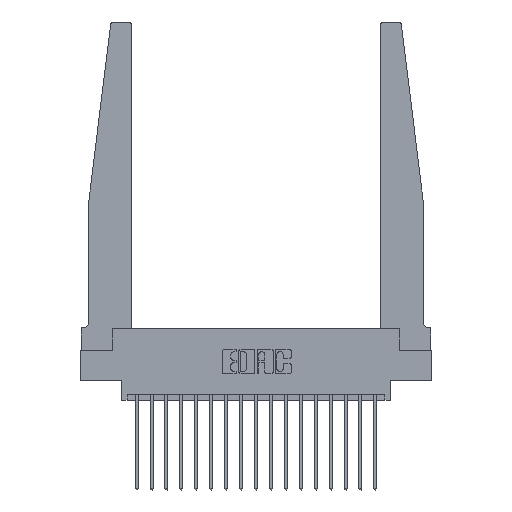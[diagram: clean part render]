
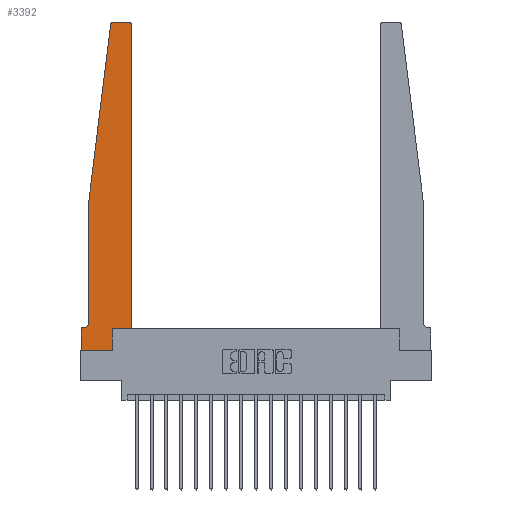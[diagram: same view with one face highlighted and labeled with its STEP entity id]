
A CAD part, top view. The second image highlights one B-rep face of the part: STEP entity #3392.
In plain terms, the highlighted planar face has unit normal (0, 0, 1).
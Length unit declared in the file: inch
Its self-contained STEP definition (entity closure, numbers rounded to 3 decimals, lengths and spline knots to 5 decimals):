
#1297 = DIRECTION ( 'NONE',  ( 0., 0., -1. ) ) ;
#1470 = VERTEX_POINT ( 'NONE', #15704 ) ;
#1640 = VECTOR ( 'NONE', #2279, 39.37008 ) ;
#1730 = DIRECTION ( 'NONE',  ( 0., 0., 1. ) ) ;
#1853 = CARTESIAN_POINT ( 'NONE',  ( 0.425, 2.72, 0.37 ) ) ;
#1882 = CARTESIAN_POINT ( 'NONE',  ( 0.24675, 2.72367, 0.37 ) ) ;
#1940 = CIRCLE ( 'NONE', #12543, 0.03 ) ;
#2054 = LINE ( 'NONE', #3768, #9599 ) ;
#2268 = CARTESIAN_POINT ( 'NONE',  ( 0.25, 2.75, 0.37 ) ) ;
#2279 = DIRECTION ( 'NONE',  ( 0., -1., 0. ) ) ;
#2594 = CARTESIAN_POINT ( 'NONE',  ( 0.015, 0.2375, 0.37 ) ) ;
#3093 = ORIENTED_EDGE ( 'NONE', *, *, #6055, .T. ) ;
#3392 = ADVANCED_FACE ( 'NONE', ( #4985 ), #8127, .T. ) ;
#3506 = LINE ( 'NONE', #9547, #18701 ) ;
#3515 = ORIENTED_EDGE ( 'NONE', *, *, #8881, .T. ) ;
#3593 = ORIENTED_EDGE ( 'NONE', *, *, #10420, .T. ) ;
#3768 = CARTESIAN_POINT ( 'NONE',  ( 0.065, 1.25, 0.37 ) ) ;
#3880 = ORIENTED_EDGE ( 'NONE', *, *, #8476, .T. ) ;
#3957 = ORIENTED_EDGE ( 'NONE', *, *, #13938, .T. ) ;
#4154 = LINE ( 'NONE', #19502, #17698 ) ;
#4369 = VECTOR ( 'NONE', #11641, 39.37008 ) ;
#4474 = AXIS2_PLACEMENT_3D ( 'NONE', #18731, #5181, #8225 ) ;
#4568 = EDGE_CURVE ( 'NONE', #5965, #17212, #12161, .T. ) ;
#4656 = DIRECTION ( 'NONE',  ( 1., 0., 0. ) ) ;
#4985 = FACE_OUTER_BOUND ( 'NONE', #17135, .T. ) ;
#5181 = DIRECTION ( 'NONE',  ( 0., 0., 1. ) ) ;
#5259 = VECTOR ( 'NONE', #18855, 39.37008 ) ;
#5777 = EDGE_CURVE ( 'NONE', #17212, #12050, #10070, .T. ) ;
#5862 = EDGE_CURVE ( 'NONE', #6694, #8320, #12257, .T. ) ;
#5960 = DIRECTION ( 'NONE',  ( 0., 1., 0. ) ) ;
#5965 = VERTEX_POINT ( 'NONE', #16452 ) ;
#6055 = EDGE_CURVE ( 'NONE', #19147, #15143, #11442, .T. ) ;
#6057 = VERTEX_POINT ( 'NONE', #19154 ) ;
#6172 = CARTESIAN_POINT ( 'NONE',  ( 0.27653, 2.72, 0.37 ) ) ;
#6395 = CARTESIAN_POINT ( 'NONE',  ( 0.27653, 2.75, 0.37 ) ) ;
#6694 = VERTEX_POINT ( 'NONE', #10810 ) ;
#7684 = AXIS2_PLACEMENT_3D ( 'NONE', #2594, #1297, #10577 ) ;
#8044 = CARTESIAN_POINT ( 'NONE',  ( 0.2605, 0., 0.37 ) ) ;
#8127 = PLANE ( 'NONE',  #4474 ) ;
#8225 = DIRECTION ( 'NONE',  ( 1., 0., 0. ) ) ;
#8231 = EDGE_CURVE ( 'NONE', #12050, #6694, #3506, .T. ) ;
#8309 = VERTEX_POINT ( 'NONE', #1882 ) ;
#8320 = VERTEX_POINT ( 'NONE', #8044 ) ;
#8322 = DIRECTION ( 'NONE',  ( -0.122, -0.992, 0. ) ) ;
#8476 = EDGE_CURVE ( 'NONE', #18237, #12462, #11435, .T. ) ;
#8881 = EDGE_CURVE ( 'NONE', #8309, #1470, #2054, .T. ) ;
#9091 = CARTESIAN_POINT ( 'NONE',  ( 0.395, 2.72, 0.37 ) ) ;
#9096 = EDGE_CURVE ( 'NONE', #15143, #18237, #16633, .T. ) ;
#9390 = DIRECTION ( 'NONE',  ( 1., 0., 0. ) ) ;
#9547 = CARTESIAN_POINT ( 'NONE',  ( 0., 0., 0.37 ) ) ;
#9599 = VECTOR ( 'NONE', #8322, 39.37008 ) ;
#9853 = LINE ( 'NONE', #17757, #1640 ) ;
#9948 = CARTESIAN_POINT ( 'NONE',  ( 0.425, 0.18, 0.37 ) ) ;
#10070 = LINE ( 'NONE', #13245, #13059 ) ;
#10327 = CARTESIAN_POINT ( 'NONE',  ( 0.425, 0.18, 0.37 ) ) ;
#10420 = EDGE_CURVE ( 'NONE', #12462, #8309, #1940, .T. ) ;
#10433 = LINE ( 'NONE', #12212, #14148 ) ;
#10577 = DIRECTION ( 'NONE',  ( -1., 0., 0. ) ) ;
#10810 = CARTESIAN_POINT ( 'NONE',  ( 0., 0., 0.37 ) ) ;
#10964 = ORIENTED_EDGE ( 'NONE', *, *, #5862, .T. ) ;
#11033 = CARTESIAN_POINT ( 'NONE',  ( 0., 0.1875, 0.37 ) ) ;
#11435 = LINE ( 'NONE', #2268, #5259 ) ;
#11442 = LINE ( 'NONE', #9948, #4369 ) ;
#11496 = ORIENTED_EDGE ( 'NONE', *, *, #11743, .T. ) ;
#11641 = DIRECTION ( 'NONE',  ( 0., 1., 0. ) ) ;
#11743 = EDGE_CURVE ( 'NONE', #1470, #5965, #9853, .T. ) ;
#12050 = VERTEX_POINT ( 'NONE', #11033 ) ;
#12161 = CIRCLE ( 'NONE', #7684, 0.05 ) ;
#12168 = ORIENTED_EDGE ( 'NONE', *, *, #5777, .T. ) ;
#12212 = CARTESIAN_POINT ( 'NONE',  ( 0.425, 0.18, 0.37 ) ) ;
#12257 = LINE ( 'NONE', #16554, #17234 ) ;
#12462 = VERTEX_POINT ( 'NONE', #6395 ) ;
#12543 = AXIS2_PLACEMENT_3D ( 'NONE', #6172, #1730, #9390 ) ;
#13059 = VECTOR ( 'NONE', #16356, 39.37008 ) ;
#13245 = CARTESIAN_POINT ( 'NONE',  ( 0.065, 0.1875, 0.37 ) ) ;
#13507 = EDGE_CURVE ( 'NONE', #6057, #19147, #10433, .T. ) ;
#13938 = EDGE_CURVE ( 'NONE', #8320, #6057, #4154, .T. ) ;
#14148 = VECTOR ( 'NONE', #16614, 39.37008 ) ;
#14404 = ORIENTED_EDGE ( 'NONE', *, *, #8231, .T. ) ;
#15143 = VERTEX_POINT ( 'NONE', #1853 ) ;
#15704 = CARTESIAN_POINT ( 'NONE',  ( 0.065, 1.25, 0.37 ) ) ;
#16356 = DIRECTION ( 'NONE',  ( -1., 0., 0. ) ) ;
#16452 = CARTESIAN_POINT ( 'NONE',  ( 0.065, 0.2375, 0.37 ) ) ;
#16554 = CARTESIAN_POINT ( 'NONE',  ( 0., 0., 0.37 ) ) ;
#16614 = DIRECTION ( 'NONE',  ( 1., 0., 0. ) ) ;
#16633 = CIRCLE ( 'NONE', #19201, 0.03 ) ;
#16834 = ORIENTED_EDGE ( 'NONE', *, *, #4568, .T. ) ;
#17076 = CARTESIAN_POINT ( 'NONE',  ( 0.015, 0.1875, 0.37 ) ) ;
#17135 = EDGE_LOOP ( 'NONE', ( #3880, #3593, #3515, #11496, #16834, #12168, #14404, #10964, #3957, #18546, #3093, #19247 ) ) ;
#17150 = DIRECTION ( 'NONE',  ( 0., -1., 0. ) ) ;
#17212 = VERTEX_POINT ( 'NONE', #17076 ) ;
#17234 = VECTOR ( 'NONE', #19762, 39.37008 ) ;
#17698 = VECTOR ( 'NONE', #5960, 39.37008 ) ;
#17757 = CARTESIAN_POINT ( 'NONE',  ( 0.065, 1.25, 0.37 ) ) ;
#18237 = VERTEX_POINT ( 'NONE', #19784 ) ;
#18302 = DIRECTION ( 'NONE',  ( 0., 0., 1. ) ) ;
#18546 = ORIENTED_EDGE ( 'NONE', *, *, #13507, .T. ) ;
#18701 = VECTOR ( 'NONE', #17150, 39.37008 ) ;
#18731 = CARTESIAN_POINT ( 'NONE',  ( 0., 0.1875, 0.37 ) ) ;
#18855 = DIRECTION ( 'NONE',  ( -1., 0., 0. ) ) ;
#19147 = VERTEX_POINT ( 'NONE', #10327 ) ;
#19154 = CARTESIAN_POINT ( 'NONE',  ( 0.2605, 0.18, 0.37 ) ) ;
#19201 = AXIS2_PLACEMENT_3D ( 'NONE', #9091, #18302, #4656 ) ;
#19247 = ORIENTED_EDGE ( 'NONE', *, *, #9096, .T. ) ;
#19502 = CARTESIAN_POINT ( 'NONE',  ( 0.2605, 0.18, 0.37 ) ) ;
#19762 = DIRECTION ( 'NONE',  ( 1., 0., 0. ) ) ;
#19784 = CARTESIAN_POINT ( 'NONE',  ( 0.395, 2.75, 0.37 ) ) ;
